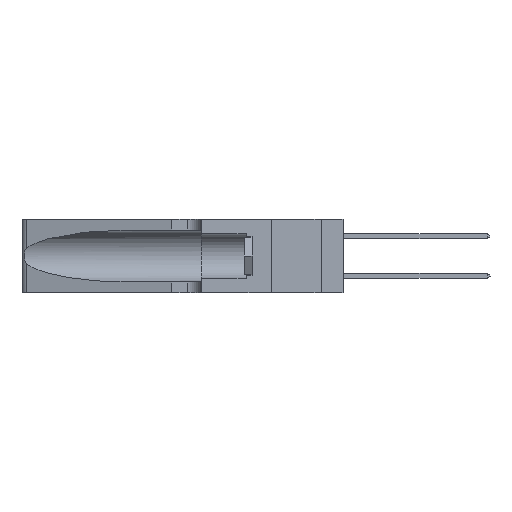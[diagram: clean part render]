
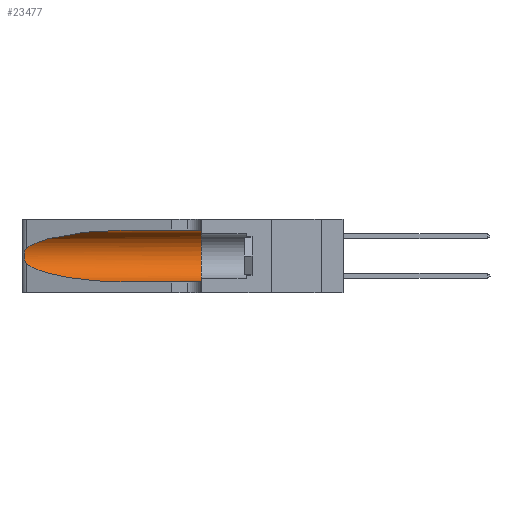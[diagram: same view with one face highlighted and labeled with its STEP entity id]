
A CAD part, left-side view. The second image highlights one B-rep face of the part: STEP entity #23477.
In plain terms, the highlighted cylindrical face has radius 3.308 mm (diameter 6.617 mm), a partial arc.
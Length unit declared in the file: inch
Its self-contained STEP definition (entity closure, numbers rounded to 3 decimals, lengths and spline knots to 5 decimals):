
#52 = VERTEX_POINT ( 'NONE', #2061 ) ;
#2061 = CARTESIAN_POINT ( 'NONE',  ( 0.25487, 1.22718, 0.22369 ) ) ;
#3204 = EDGE_CURVE ( 'NONE', #15980, #14456, #8149, .T. ) ;
#3382 = CARTESIAN_POINT ( 'NONE',  ( 0.25639, 1.23186, 0.15144 ) ) ;
#3480 = EDGE_CURVE ( 'NONE', #52, #4135, #23261, .T. ) ;
#3538 = DIRECTION ( 'NONE',  ( 0., 1., 0. ) ) ;
#4135 = VERTEX_POINT ( 'NONE', #22047 ) ;
#4817 =( BOUNDED_CURVE ( )  B_SPLINE_CURVE ( 3, ( #8615, #16428, #23603, #12393 ),
 .UNSPECIFIED., .F., .F. ) 
 B_SPLINE_CURVE_WITH_KNOTS ( ( 4, 4 ),
 ( 1.5708, 2.84003 ),
 .UNSPECIFIED. ) 
 CURVE ( )  GEOMETRIC_REPRESENTATION_ITEM ( )  RATIONAL_B_SPLINE_CURVE ( ( 1., 0.87, 0.87, 1. ) ) 
 REPRESENTATION_ITEM ( '' )  );
#4994 = VERTEX_POINT ( 'NONE', #7954 ) ;
#5662 = DIRECTION ( 'NONE',  ( 0., 0., 1. ) ) ;
#5742 = CARTESIAN_POINT ( 'NONE',  ( 0.1305, 0.35, 0.185 ) ) ;
#6116 = LINE ( 'NONE', #14184, #16112 ) ;
#6893 = CARTESIAN_POINT ( 'NONE',  ( 0.25639, 1.23184, 0.21858 ) ) ;
#6974 = CARTESIAN_POINT ( 'NONE',  ( 0.26018, 1.23835, 0.19895 ) ) ;
#7059 = ORIENTED_EDGE ( 'NONE', *, *, #17117, .T. ) ;
#7060 = CARTESIAN_POINT ( 'NONE',  ( 0.26017, 1.23833, 0.17102 ) ) ;
#7312 = EDGE_CURVE ( 'NONE', #4994, #14456, #22716, .T. ) ;
#7915 = AXIS2_PLACEMENT_3D ( 'NONE', #5742, #3538, #5662 ) ;
#7954 = CARTESIAN_POINT ( 'NONE',  ( 0.1305, 0.35, 0.31525 ) ) ;
#8144 = CYLINDRICAL_SURFACE ( 'NONE', #23990, 0.13025 ) ;
#8149 = LINE ( 'NONE', #23757, #22212 ) ;
#8615 = CARTESIAN_POINT ( 'NONE',  ( 0.1305, 0.72297, 0.31525 ) ) ;
#8761 = CARTESIAN_POINT ( 'NONE',  ( 0.25787, 1.23484, 0.2124 ) ) ;
#10349 = CARTESIAN_POINT ( 'NONE',  ( 0.1305, 0.35, 0.05475 ) ) ;
#10610 = EDGE_CURVE ( 'NONE', #4135, #15980, #10967, .T. ) ;
#10751 = CARTESIAN_POINT ( 'NONE',  ( 0.26075, 1.23896, 0.19203 ) ) ;
#10831 = CARTESIAN_POINT ( 'NONE',  ( 0.25789, 1.23486, 0.15765 ) ) ;
#10967 =( BOUNDED_CURVE ( )  B_SPLINE_CURVE ( 3, ( #21389, #19510, #21312, #19358 ),
 .UNSPECIFIED., .F., .T. ) 
 B_SPLINE_CURVE_WITH_KNOTS ( ( 4, 4 ),
 ( 3.44316, 4.71239 ),
 .UNSPECIFIED. ) 
 CURVE ( )  GEOMETRIC_REPRESENTATION_ITEM ( )  RATIONAL_B_SPLINE_CURVE ( ( 1., 0.87, 0.87, 1. ) ) 
 REPRESENTATION_ITEM ( '' )  );
#10986 = ORIENTED_EDGE ( 'NONE', *, *, #22531, .F. ) ;
#12393 = CARTESIAN_POINT ( 'NONE',  ( 0.25487, 1.22718, 0.22369 ) ) ;
#12543 = FACE_OUTER_BOUND ( 'NONE', #21762, .T. ) ;
#12624 = CARTESIAN_POINT ( 'NONE',  ( 0.25856, 1.23593, 0.16098 ) ) ;
#12716 = CARTESIAN_POINT ( 'NONE',  ( 0.25487, 1.22718, 0.14631 ) ) ;
#13366 = CARTESIAN_POINT ( 'NONE',  ( 0.1305, 0.72297, 0.31525 ) ) ;
#13643 = ORIENTED_EDGE ( 'NONE', *, *, #3204, .T. ) ;
#14184 = CARTESIAN_POINT ( 'NONE',  ( 0.1305, 1.61858, 0.31525 ) ) ;
#14372 = CARTESIAN_POINT ( 'NONE',  ( 0.25487, 1.22718, 0.22369 ) ) ;
#14456 = VERTEX_POINT ( 'NONE', #10349 ) ;
#15980 = VERTEX_POINT ( 'NONE', #20146 ) ;
#16039 = ORIENTED_EDGE ( 'NONE', *, *, #3480, .T. ) ;
#16112 = VECTOR ( 'NONE', #19394, 39.37008 ) ;
#16247 = CARTESIAN_POINT ( 'NONE',  ( 0.25555, 1.22994, 0.2215 ) ) ;
#16332 = CARTESIAN_POINT ( 'NONE',  ( 0.25854, 1.2359, 0.20912 ) ) ;
#16361 = DIRECTION ( 'NONE',  ( 0., -1., 0. ) ) ;
#16407 = ORIENTED_EDGE ( 'NONE', *, *, #7312, .F. ) ;
#16428 = CARTESIAN_POINT ( 'NONE',  ( 0.18966, 0.96281, 0.31525 ) ) ;
#16522 = CARTESIAN_POINT ( 'NONE',  ( 0.1305, 1.61858, 0.185 ) ) ;
#17117 = EDGE_CURVE ( 'NONE', #17354, #52, #4817, .T. ) ;
#17354 = VERTEX_POINT ( 'NONE', #13366 ) ;
#18216 = ORIENTED_EDGE ( 'NONE', *, *, #10610, .T. ) ;
#19358 = CARTESIAN_POINT ( 'NONE',  ( 0.1305, 0.72297, 0.05475 ) ) ;
#19394 = DIRECTION ( 'NONE',  ( 0., -1., 0. ) ) ;
#19510 = CARTESIAN_POINT ( 'NONE',  ( 0.2373, 1.15595, 0.08982 ) ) ;
#20066 = DIRECTION ( 'NONE',  ( 0., -1., 0. ) ) ;
#20146 = CARTESIAN_POINT ( 'NONE',  ( 0.1305, 0.72297, 0.05475 ) ) ;
#20168 = DIRECTION ( 'NONE',  ( 0., 0., -1. ) ) ;
#21312 = CARTESIAN_POINT ( 'NONE',  ( 0.18966, 0.96281, 0.05475 ) ) ;
#21389 = CARTESIAN_POINT ( 'NONE',  ( 0.25487, 1.22718, 0.14631 ) ) ;
#21762 = EDGE_LOOP ( 'NONE', ( #7059, #16039, #18216, #13643, #16407, #10986 ) ) ;
#22047 = CARTESIAN_POINT ( 'NONE',  ( 0.25487, 1.22718, 0.14631 ) ) ;
#22212 = VECTOR ( 'NONE', #20066, 39.37008 ) ;
#22531 = EDGE_CURVE ( 'NONE', #17354, #4994, #6116, .T. ) ;
#22716 = CIRCLE ( 'NONE', #7915, 0.13025 ) ;
#23261 = B_SPLINE_CURVE_WITH_KNOTS ( 'NONE', 3,
 ( #14372, #16247, #6893, #8761, #16332, #6974, #10751, #23839, #7060, #12624, #10831, #3382, #23920, #12716 ),
 .UNSPECIFIED., .F., .F.,
 ( 4, 2, 2, 2, 2, 2, 4 ),
 ( 0., 0.00027, 0.00053, 0.00107, 0.0016, 0.00187, 0.00214 ),
 .UNSPECIFIED. ) ;
#23477 = ADVANCED_FACE ( 'NONE', ( #12543 ), #8144, .F. ) ;
#23603 = CARTESIAN_POINT ( 'NONE',  ( 0.2373, 1.15595, 0.28018 ) ) ;
#23757 = CARTESIAN_POINT ( 'NONE',  ( 0.1305, 1.61858, 0.05475 ) ) ;
#23839 = CARTESIAN_POINT ( 'NONE',  ( 0.26075, 1.23896, 0.178 ) ) ;
#23920 = CARTESIAN_POINT ( 'NONE',  ( 0.25555, 1.22993, 0.14849 ) ) ;
#23990 = AXIS2_PLACEMENT_3D ( 'NONE', #16522, #16361, #20168 ) ;
